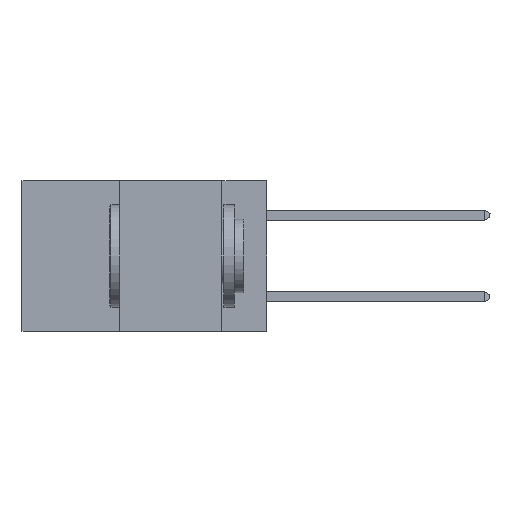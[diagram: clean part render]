
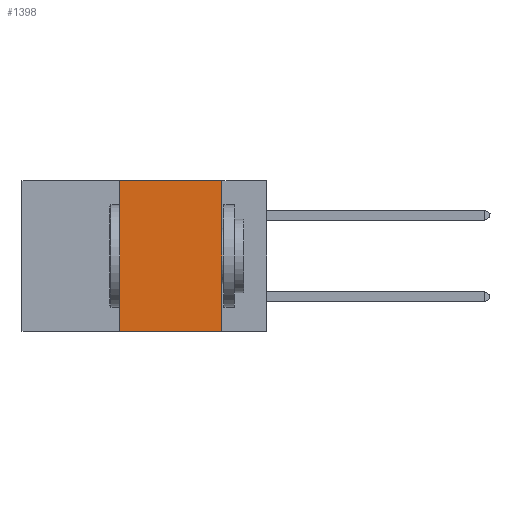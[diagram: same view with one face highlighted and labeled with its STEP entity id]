
A CAD part, left-side view. The second image highlights one B-rep face of the part: STEP entity #1398.
In plain terms, the highlighted planar face has unit normal (-1, 0, 0).
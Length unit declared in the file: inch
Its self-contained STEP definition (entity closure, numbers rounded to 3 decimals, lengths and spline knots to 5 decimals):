
#404 = DIRECTION ( 'NONE',  ( 0., -1., 0. ) ) ;
#586 = VERTEX_POINT ( 'NONE', #2175 ) ;
#798 = ORIENTED_EDGE ( 'NONE', *, *, #3045, .F. ) ;
#1059 = CARTESIAN_POINT ( 'NONE',  ( 0., 0.11, 0. ) ) ;
#1398 = ADVANCED_FACE ( 'NONE', ( #7660 ), #9406, .F. ) ;
#1547 = CARTESIAN_POINT ( 'NONE',  ( 0., 0.11, -0.37 ) ) ;
#1968 = EDGE_LOOP ( 'NONE', ( #798, #6814, #5864, #3100 ) ) ;
#2175 = CARTESIAN_POINT ( 'NONE',  ( 0., 0.36, -0.37 ) ) ;
#2478 = VERTEX_POINT ( 'NONE', #1547 ) ;
#3045 = EDGE_CURVE ( 'NONE', #6370, #2478, #3498, .T. ) ;
#3100 = ORIENTED_EDGE ( 'NONE', *, *, #5386, .T. ) ;
#3197 = EDGE_CURVE ( 'NONE', #586, #5225, #8315, .T. ) ;
#3498 = LINE ( 'NONE', #7259, #4415 ) ;
#3551 = VECTOR ( 'NONE', #9557, 39.37008 ) ;
#4415 = VECTOR ( 'NONE', #5418, 39.37008 ) ;
#4470 = LINE ( 'NONE', #7227, #3551 ) ;
#4478 = AXIS2_PLACEMENT_3D ( 'NONE', #5944, #10983, #7570 ) ;
#5225 = VERTEX_POINT ( 'NONE', #6821 ) ;
#5386 = EDGE_CURVE ( 'NONE', #586, #2478, #10803, .T. ) ;
#5418 = DIRECTION ( 'NONE',  ( 0., 0., -1. ) ) ;
#5864 = ORIENTED_EDGE ( 'NONE', *, *, #3197, .F. ) ;
#5944 = CARTESIAN_POINT ( 'NONE',  ( 0., 0.6, 0. ) ) ;
#6244 = DIRECTION ( 'NONE',  ( 0., 0., 1. ) ) ;
#6355 = EDGE_CURVE ( 'NONE', #5225, #6370, #4470, .T. ) ;
#6359 = CARTESIAN_POINT ( 'NONE',  ( 0., 0.6, -0.37 ) ) ;
#6370 = VERTEX_POINT ( 'NONE', #1059 ) ;
#6814 = ORIENTED_EDGE ( 'NONE', *, *, #6355, .F. ) ;
#6821 = CARTESIAN_POINT ( 'NONE',  ( 0., 0.36, 0. ) ) ;
#7227 = CARTESIAN_POINT ( 'NONE',  ( 0., 0.6, 0. ) ) ;
#7259 = CARTESIAN_POINT ( 'NONE',  ( 0., 0.11, 0. ) ) ;
#7570 = DIRECTION ( 'NONE',  ( 0., 0., -1. ) ) ;
#7660 = FACE_OUTER_BOUND ( 'NONE', #1968, .T. ) ;
#8315 = LINE ( 'NONE', #8819, #10309 ) ;
#8819 = CARTESIAN_POINT ( 'NONE',  ( 0., 0.36, 0. ) ) ;
#9406 = PLANE ( 'NONE',  #4478 ) ;
#9557 = DIRECTION ( 'NONE',  ( 0., -1., 0. ) ) ;
#10309 = VECTOR ( 'NONE', #6244, 39.37008 ) ;
#10393 = VECTOR ( 'NONE', #404, 39.37008 ) ;
#10803 = LINE ( 'NONE', #6359, #10393 ) ;
#10983 = DIRECTION ( 'NONE',  ( 1., 0., 0. ) ) ;
